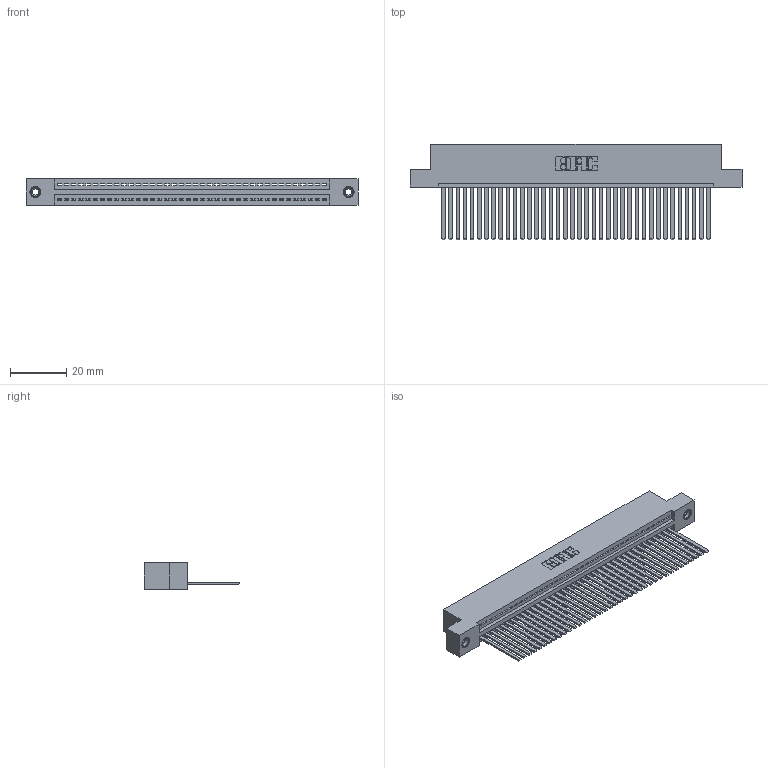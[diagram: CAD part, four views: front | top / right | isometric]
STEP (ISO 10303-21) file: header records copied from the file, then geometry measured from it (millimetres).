
FILE_DESCRIPTION (( 'STEP AP203' ), '1' );
FILE_NAME ('395-038-544-108.STEP', '2018-11-14T05:10:47', ( '' ), ( '' ), 'SwSTEP 2.0', 'SolidWorks 2016', '' );
FILE_SCHEMA (( 'CONFIG_CONTROL_DESIGN' ));
Length unit declared in the file: inch
Products named in the file (4): 395-038-544-108; 345-292-001_345-293-144; 345 Part_Flush Mounting Lugs - 0.156 Dia-TI; 345-250-001_345-250-003-102
Assembly tree (41 placements, depth 2):
  395-038-544-108
    345 Part_Flush Mounting Lugs - 0.156 Dia-TI
    345-292-001_345-293-144  x38
    345-250-001_345-250-003-102  x2
Bounding box: 117.73 x 33.96 x 9.4 mm (x, y, z)
Volume: 11582.8 mm3; surface area: 16678.5 mm2
Topology: 41 solids, 41 shells, 2162 faces, 6481 edges, 4262 vertices
Faces by surface type: plane 1480, cylinder 666, cone 12, torus 4
Entity records: 30140 total; most frequent: CARTESIAN_POINT 5201, ORIENTED_EDGE 5166, DIRECTION 4573, EDGE_CURVE 2583, LINE 2283, VECTOR 2283, VERTEX_POINT 1716, AXIS2_PLACEMENT_3D 1145
